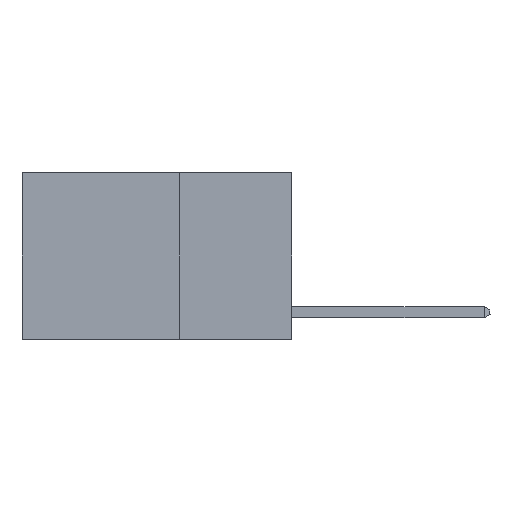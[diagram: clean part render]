
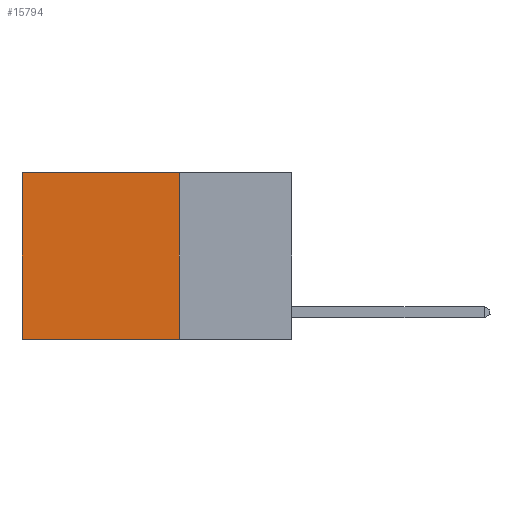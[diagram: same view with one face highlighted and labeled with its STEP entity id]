
A CAD part, left-side view. The second image highlights one B-rep face of the part: STEP entity #15794.
In plain terms, the highlighted planar face has unit normal (-1, 0, 0).
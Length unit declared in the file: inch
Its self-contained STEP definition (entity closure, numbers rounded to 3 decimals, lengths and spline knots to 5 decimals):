
#314 = DIRECTION ( 'NONE',  ( 0., 0., -1. ) ) ;
#1473 = EDGE_LOOP ( 'NONE', ( #1794, #13914, #14364, #12548 ) ) ;
#1610 = CARTESIAN_POINT ( 'NONE',  ( 0.2625, 0.25, 0. ) ) ;
#1639 = VECTOR ( 'NONE', #8672, 39.37008 ) ;
#1657 = CARTESIAN_POINT ( 'NONE',  ( 0.2625, 0.6, 0. ) ) ;
#1733 = CARTESIAN_POINT ( 'NONE',  ( 0.2625, 0.25, 0. ) ) ;
#1794 = ORIENTED_EDGE ( 'NONE', *, *, #11784, .T. ) ;
#1996 = VERTEX_POINT ( 'NONE', #10478 ) ;
#2577 = EDGE_CURVE ( 'NONE', #14985, #1996, #3741, .T. ) ;
#2946 = DIRECTION ( 'NONE',  ( 0., 0., -1. ) ) ;
#2952 = CARTESIAN_POINT ( 'NONE',  ( 0.2625, 0.25, -0.37 ) ) ;
#3317 = VECTOR ( 'NONE', #15680, 39.37008 ) ;
#3741 = LINE ( 'NONE', #6618, #3317 ) ;
#4163 = VERTEX_POINT ( 'NONE', #11599 ) ;
#4761 = LINE ( 'NONE', #1657, #14720 ) ;
#5324 = VERTEX_POINT ( 'NONE', #11229 ) ;
#6618 = CARTESIAN_POINT ( 'NONE',  ( 0.2625, 0.25, 0. ) ) ;
#7282 = EDGE_CURVE ( 'NONE', #1996, #4163, #12007, .T. ) ;
#8294 = DIRECTION ( 'NONE',  ( 0., 1., 0. ) ) ;
#8554 = VECTOR ( 'NONE', #8294, 39.37008 ) ;
#8672 = DIRECTION ( 'NONE',  ( 0., 1., 0. ) ) ;
#9304 = AXIS2_PLACEMENT_3D ( 'NONE', #1610, #10826, #2946 ) ;
#10478 = CARTESIAN_POINT ( 'NONE',  ( 0.2625, 0.25, -0.37 ) ) ;
#10826 = DIRECTION ( 'NONE',  ( 1., 0., 0. ) ) ;
#11229 = CARTESIAN_POINT ( 'NONE',  ( 0.2625, 0.6, 0. ) ) ;
#11599 = CARTESIAN_POINT ( 'NONE',  ( 0.2625, 0.6, -0.37 ) ) ;
#11784 = EDGE_CURVE ( 'NONE', #5324, #4163, #4761, .T. ) ;
#12007 = LINE ( 'NONE', #2952, #8554 ) ;
#12543 = CARTESIAN_POINT ( 'NONE',  ( 0.2625, 0.25, 0. ) ) ;
#12548 = ORIENTED_EDGE ( 'NONE', *, *, #15173, .T. ) ;
#12549 = LINE ( 'NONE', #12543, #1639 ) ;
#13368 = PLANE ( 'NONE',  #9304 ) ;
#13914 = ORIENTED_EDGE ( 'NONE', *, *, #7282, .F. ) ;
#14364 = ORIENTED_EDGE ( 'NONE', *, *, #2577, .F. ) ;
#14720 = VECTOR ( 'NONE', #314, 39.37008 ) ;
#14985 = VERTEX_POINT ( 'NONE', #1733 ) ;
#15173 = EDGE_CURVE ( 'NONE', #14985, #5324, #12549, .T. ) ;
#15289 = FACE_OUTER_BOUND ( 'NONE', #1473, .T. ) ;
#15680 = DIRECTION ( 'NONE',  ( 0., 0., -1. ) ) ;
#15794 = ADVANCED_FACE ( 'NONE', ( #15289 ), #13368, .F. ) ;
